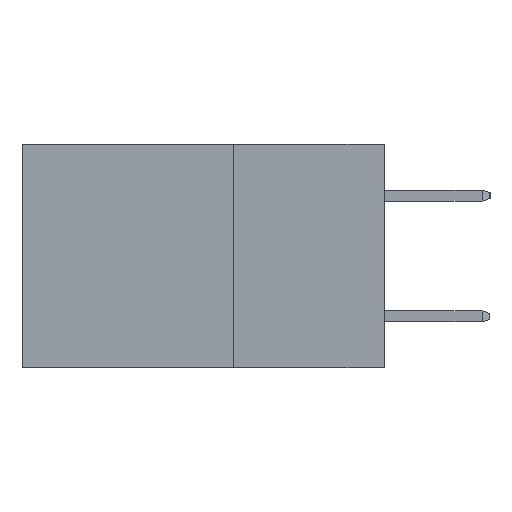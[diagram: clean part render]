
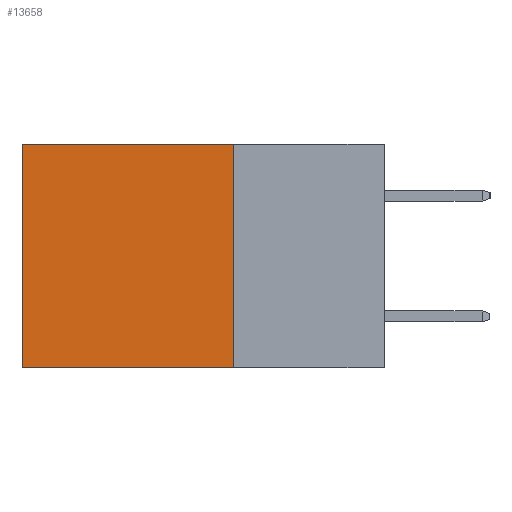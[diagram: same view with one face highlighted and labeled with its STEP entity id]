
A CAD part, left-side view. The second image highlights one B-rep face of the part: STEP entity #13658.
In plain terms, the highlighted planar face has unit normal (-1, 0, 0).
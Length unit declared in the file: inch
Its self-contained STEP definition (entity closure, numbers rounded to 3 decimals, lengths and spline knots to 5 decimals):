
#886 = VERTEX_POINT ( 'NONE', #2892 ) ;
#1030 = LINE ( 'NONE', #9357, #6578 ) ;
#1293 = ORIENTED_EDGE ( 'NONE', *, *, #7950, .T. ) ;
#1652 = VERTEX_POINT ( 'NONE', #4302 ) ;
#1706 = EDGE_CURVE ( 'NONE', #4282, #12443, #5414, .T. ) ;
#2067 = EDGE_LOOP ( 'NONE', ( #1293, #9027, #6341, #2888 ) ) ;
#2291 = DIRECTION ( 'NONE',  ( 0., 1., 0. ) ) ;
#2819 = CARTESIAN_POINT ( 'NONE',  ( 0.298, 0.25, -0.37 ) ) ;
#2888 = ORIENTED_EDGE ( 'NONE', *, *, #4721, .T. ) ;
#2892 = CARTESIAN_POINT ( 'NONE',  ( 0.298, 0.6, 0. ) ) ;
#3011 = VECTOR ( 'NONE', #2291, 39.37008 ) ;
#3386 = LINE ( 'NONE', #13920, #3011 ) ;
#4282 = VERTEX_POINT ( 'NONE', #13070 ) ;
#4302 = CARTESIAN_POINT ( 'NONE',  ( 0.298, 0.6, -0.37 ) ) ;
#4390 = VECTOR ( 'NONE', #12874, 39.37008 ) ;
#4451 = DIRECTION ( 'NONE',  ( 0., 1., 0. ) ) ;
#4721 = EDGE_CURVE ( 'NONE', #4282, #886, #1030, .T. ) ;
#5225 = CARTESIAN_POINT ( 'NONE',  ( 0.298, 0.25, 0. ) ) ;
#5414 = LINE ( 'NONE', #10916, #4390 ) ;
#6262 = DIRECTION ( 'NONE',  ( 0., 0., -1. ) ) ;
#6271 = DIRECTION ( 'NONE',  ( 0., 0., -1. ) ) ;
#6341 = ORIENTED_EDGE ( 'NONE', *, *, #1706, .F. ) ;
#6578 = VECTOR ( 'NONE', #4451, 39.37008 ) ;
#7107 = FACE_OUTER_BOUND ( 'NONE', #2067, .T. ) ;
#7436 = VECTOR ( 'NONE', #6271, 39.37008 ) ;
#7473 = AXIS2_PLACEMENT_3D ( 'NONE', #5225, #12444, #6262 ) ;
#7776 = LINE ( 'NONE', #12453, #7436 ) ;
#7950 = EDGE_CURVE ( 'NONE', #886, #1652, #7776, .T. ) ;
#9027 = ORIENTED_EDGE ( 'NONE', *, *, #13500, .F. ) ;
#9357 = CARTESIAN_POINT ( 'NONE',  ( 0.298, 0.25, 0. ) ) ;
#10916 = CARTESIAN_POINT ( 'NONE',  ( 0.298, 0.25, 0. ) ) ;
#11460 = PLANE ( 'NONE',  #7473 ) ;
#12443 = VERTEX_POINT ( 'NONE', #2819 ) ;
#12444 = DIRECTION ( 'NONE',  ( 1., 0., 0. ) ) ;
#12453 = CARTESIAN_POINT ( 'NONE',  ( 0.298, 0.6, 0. ) ) ;
#12874 = DIRECTION ( 'NONE',  ( 0., 0., -1. ) ) ;
#13070 = CARTESIAN_POINT ( 'NONE',  ( 0.298, 0.25, 0. ) ) ;
#13500 = EDGE_CURVE ( 'NONE', #12443, #1652, #3386, .T. ) ;
#13658 = ADVANCED_FACE ( 'NONE', ( #7107 ), #11460, .F. ) ;
#13920 = CARTESIAN_POINT ( 'NONE',  ( 0.298, 0.25, -0.37 ) ) ;
